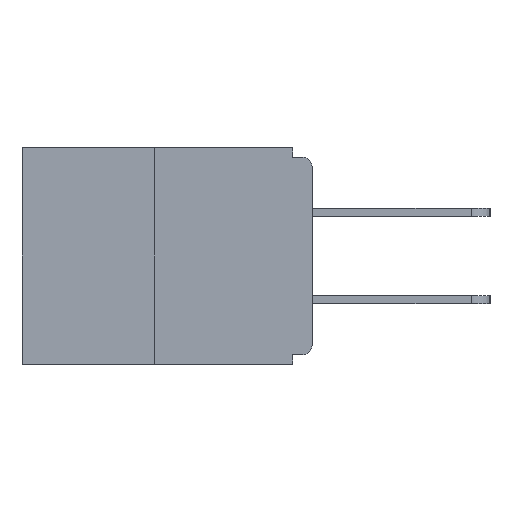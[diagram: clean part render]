
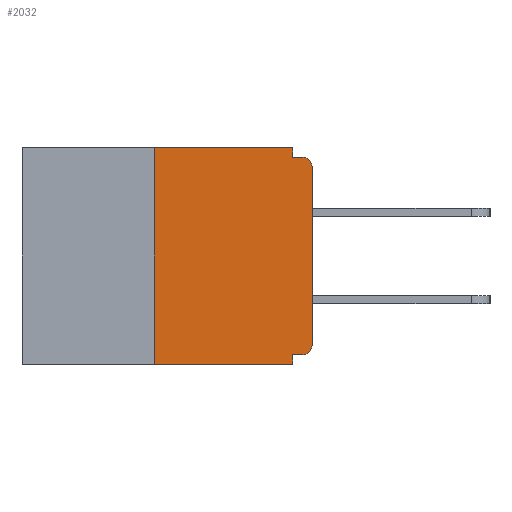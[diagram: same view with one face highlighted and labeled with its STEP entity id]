
A CAD part, left-side view. The second image highlights one B-rep face of the part: STEP entity #2032.
In plain terms, the highlighted planar face has unit normal (-1, 0, 0).
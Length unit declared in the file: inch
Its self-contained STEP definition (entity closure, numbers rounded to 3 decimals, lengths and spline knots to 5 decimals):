
#479 = DIRECTION ( 'NONE',  ( 0., 0., -1. ) ) ;
#513 = VERTEX_POINT ( 'NONE', #11628 ) ;
#605 = DIRECTION ( 'NONE',  ( 0., 0., 1. ) ) ;
#724 = LINE ( 'NONE', #12405, #10970 ) ;
#796 = CARTESIAN_POINT ( 'NONE',  ( 0., 0.031, 0. ) ) ;
#913 = DIRECTION ( 'NONE',  ( 0., 0., -1. ) ) ;
#975 = CARTESIAN_POINT ( 'NONE',  ( 0., 0.015, -0.03 ) ) ;
#1025 = VERTEX_POINT ( 'NONE', #1057 ) ;
#1057 = CARTESIAN_POINT ( 'NONE',  ( 0., 0.015, -0.328 ) ) ;
#1177 = CARTESIAN_POINT ( 'NONE',  ( 0., 0.46, 0. ) ) ;
#1398 = DIRECTION ( 'NONE',  ( 0., 1., 0. ) ) ;
#1541 = ORIENTED_EDGE ( 'NONE', *, *, #8188, .F. ) ;
#1742 = AXIS2_PLACEMENT_3D ( 'NONE', #8791, #18470, #5731 ) ;
#2032 = ADVANCED_FACE ( 'NONE', ( #7116 ), #2033, .F. ) ;
#2033 = PLANE ( 'NONE',  #4410 ) ;
#2093 = CARTESIAN_POINT ( 'NONE',  ( 0., 0.46, 0. ) ) ;
#2352 = ORIENTED_EDGE ( 'NONE', *, *, #5366, .T. ) ;
#2412 = CARTESIAN_POINT ( 'NONE',  ( 0., 0.031, -0.343 ) ) ;
#2791 = DIRECTION ( 'NONE',  ( 0., -1., 0. ) ) ;
#3013 = VECTOR ( 'NONE', #1398, 39.37008 ) ;
#3071 = VERTEX_POINT ( 'NONE', #19486 ) ;
#3235 = VECTOR ( 'NONE', #10231, 39.37008 ) ;
#3319 = CARTESIAN_POINT ( 'NONE',  ( 0., 0., 0. ) ) ;
#3462 = VERTEX_POINT ( 'NONE', #4979 ) ;
#3570 = LINE ( 'NONE', #1177, #5323 ) ;
#3586 = VERTEX_POINT ( 'NONE', #10034 ) ;
#3759 = CARTESIAN_POINT ( 'NONE',  ( 0., 0.25, 0. ) ) ;
#4294 = LINE ( 'NONE', #15074, #19100 ) ;
#4410 = AXIS2_PLACEMENT_3D ( 'NONE', #2093, #19481, #479 ) ;
#4521 = EDGE_CURVE ( 'NONE', #513, #5991, #17843, .T. ) ;
#4764 = LINE ( 'NONE', #9313, #3013 ) ;
#4979 = CARTESIAN_POINT ( 'NONE',  ( 0., 0.25, -0.343 ) ) ;
#5235 = CARTESIAN_POINT ( 'NONE',  ( 0., 0.031, -0.328 ) ) ;
#5284 = VECTOR ( 'NONE', #6730, 39.37008 ) ;
#5323 = VECTOR ( 'NONE', #5832, 39.37008 ) ;
#5366 = EDGE_CURVE ( 'NONE', #3462, #3071, #724, .T. ) ;
#5731 = DIRECTION ( 'NONE',  ( 0., 0., -1. ) ) ;
#5761 = ORIENTED_EDGE ( 'NONE', *, *, #5887, .T. ) ;
#5832 = DIRECTION ( 'NONE',  ( 0., -1., 0. ) ) ;
#5887 = EDGE_CURVE ( 'NONE', #1025, #513, #7754, .T. ) ;
#5975 = ORIENTED_EDGE ( 'NONE', *, *, #4521, .T. ) ;
#5991 = VERTEX_POINT ( 'NONE', #18740 ) ;
#6020 = LINE ( 'NONE', #16334, #5284 ) ;
#6730 = DIRECTION ( 'NONE',  ( 0., -1., 0. ) ) ;
#7116 = FACE_OUTER_BOUND ( 'NONE', #8482, .T. ) ;
#7387 = EDGE_CURVE ( 'NONE', #13836, #3586, #3570, .T. ) ;
#7754 = CIRCLE ( 'NONE', #1742, 0.015 ) ;
#7964 = LINE ( 'NONE', #2412, #20004 ) ;
#8188 = EDGE_CURVE ( 'NONE', #3462, #13836, #4294, .T. ) ;
#8412 = ORIENTED_EDGE ( 'NONE', *, *, #16681, .F. ) ;
#8482 = EDGE_LOOP ( 'NONE', ( #13337, #1541, #2352, #8737, #16095, #5761, #5975, #16053, #10364, #8412 ) ) ;
#8737 = ORIENTED_EDGE ( 'NONE', *, *, #16237, .F. ) ;
#8791 = CARTESIAN_POINT ( 'NONE',  ( 0., 0.015, -0.313 ) ) ;
#8993 = EDGE_CURVE ( 'NONE', #9635, #18122, #6020, .T. ) ;
#9313 = CARTESIAN_POINT ( 'NONE',  ( 0., 0., -0.328 ) ) ;
#9317 = EDGE_CURVE ( 'NONE', #1025, #18256, #4764, .T. ) ;
#9635 = VERTEX_POINT ( 'NONE', #17216 ) ;
#10034 = CARTESIAN_POINT ( 'NONE',  ( 0., 0.031, 0. ) ) ;
#10231 = DIRECTION ( 'NONE',  ( 0., 0., -1. ) ) ;
#10364 = ORIENTED_EDGE ( 'NONE', *, *, #8993, .F. ) ;
#10937 = EDGE_CURVE ( 'NONE', #5991, #18122, #18449, .T. ) ;
#10970 = VECTOR ( 'NONE', #2791, 39.37008 ) ;
#11515 = VECTOR ( 'NONE', #15977, 39.37008 ) ;
#11628 = CARTESIAN_POINT ( 'NONE',  ( 0., 0., -0.313 ) ) ;
#12405 = CARTESIAN_POINT ( 'NONE',  ( 0., 0.46, -0.343 ) ) ;
#12965 = CARTESIAN_POINT ( 'NONE',  ( 0., 0.015, -0.015 ) ) ;
#13337 = ORIENTED_EDGE ( 'NONE', *, *, #7387, .F. ) ;
#13836 = VERTEX_POINT ( 'NONE', #3759 ) ;
#15074 = CARTESIAN_POINT ( 'NONE',  ( 0., 0.25, 0. ) ) ;
#15473 = LINE ( 'NONE', #796, #3235 ) ;
#15624 = DIRECTION ( 'NONE',  ( 0., 0., -1. ) ) ;
#15639 = AXIS2_PLACEMENT_3D ( 'NONE', #975, #17014, #15624 ) ;
#15977 = DIRECTION ( 'NONE',  ( 0., 0., 1. ) ) ;
#16053 = ORIENTED_EDGE ( 'NONE', *, *, #10937, .T. ) ;
#16095 = ORIENTED_EDGE ( 'NONE', *, *, #9317, .F. ) ;
#16237 = EDGE_CURVE ( 'NONE', #18256, #3071, #7964, .T. ) ;
#16334 = CARTESIAN_POINT ( 'NONE',  ( 0., 0., -0.015 ) ) ;
#16681 = EDGE_CURVE ( 'NONE', #3586, #9635, #15473, .T. ) ;
#17014 = DIRECTION ( 'NONE',  ( -1., 0., 0. ) ) ;
#17216 = CARTESIAN_POINT ( 'NONE',  ( 0., 0.031, -0.015 ) ) ;
#17843 = LINE ( 'NONE', #3319, #11515 ) ;
#18122 = VERTEX_POINT ( 'NONE', #12965 ) ;
#18256 = VERTEX_POINT ( 'NONE', #5235 ) ;
#18449 = CIRCLE ( 'NONE', #15639, 0.015 ) ;
#18470 = DIRECTION ( 'NONE',  ( -1., 0., 0. ) ) ;
#18740 = CARTESIAN_POINT ( 'NONE',  ( 0., 0., -0.03 ) ) ;
#19100 = VECTOR ( 'NONE', #605, 39.37008 ) ;
#19481 = DIRECTION ( 'NONE',  ( 1., 0., 0. ) ) ;
#19486 = CARTESIAN_POINT ( 'NONE',  ( 0., 0.031, -0.343 ) ) ;
#20004 = VECTOR ( 'NONE', #913, 39.37008 ) ;
